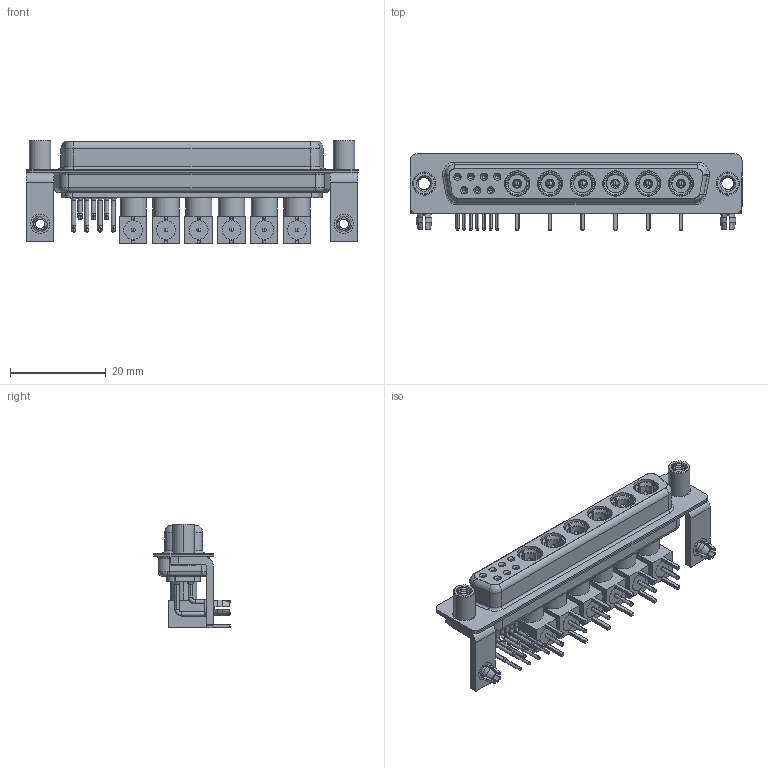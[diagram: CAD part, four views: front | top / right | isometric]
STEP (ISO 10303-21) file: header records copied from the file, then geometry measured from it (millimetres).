
FILE_DESCRIPTION (( 'STEP AP203' ), '1' );
FILE_NAME ('630-13W6240-7TD.STEP', '2022-06-03T13:02:00', ( '' ), ( '' ), 'SwSTEP 2.0', 'SolidWorks 2020', '' );
FILE_SCHEMA (( 'CONFIG_CONTROL_DESIGN' ));
Length unit declared in the file: millimetre
Products named in the file (21): Insulator RA Pin; RA Back Shell; 630Combo Contact Row 1; Pin_RA; 630Combo Shell Front_37 Contacts; Co-Ax Plug Assy_RA; Co-Ax Plug_RA PC Tail; 630Combo Shell Rear_37 Contacts; 630Combo Stabilizer Bracket; 630Combo Board Lock; Locking Collar; 630Combo Contact Row 2; 630Combo Housing_13W6; Insulator Pin_Straight PC Tail; 630Combo Threaded Standoff_D; 630-13W6240-7TD
Assembly tree (58 placements, depth 3):
  630-13W6240-7TD
    630Combo Housing_13W6
    630Combo Shell Front_37 Contacts
    630Combo Shell Rear_37 Contacts
    630Combo Stabilizer Bracket  x2
    630Combo Board Lock  x2
    630Combo Threaded Standoff_D  x2
    Co-Ax Plug Assy_RA
      Co-Ax Plug_RA PC Tail
      Insulator Pin_Straight PC Tail
      Pin_RA
      Locking Collar
      RA Back Shell
      Insulator RA Pin
    Co-Ax Plug Assy_RA
      Co-Ax Plug_RA PC Tail
      Insulator Pin_Straight PC Tail
      Pin_RA
      Locking Collar
      RA Back Shell
      Insulator RA Pin
    Co-Ax Plug Assy_RA
      Co-Ax Plug_RA PC Tail
      Insulator Pin_Straight PC Tail
      Pin_RA
      Locking Collar
      RA Back Shell
      Insulator RA Pin
    Co-Ax Plug Assy_RA
      Co-Ax Plug_RA PC Tail
      Insulator Pin_Straight PC Tail
      Pin_RA
      Locking Collar
      RA Back Shell
      Insulator RA Pin
    Co-Ax Plug Assy_RA
      Co-Ax Plug_RA PC Tail
      Insulator Pin_Straight PC Tail
      Pin_RA
      Locking Collar
      RA Back Shell
      Insulator RA Pin
    Co-Ax Plug Assy_RA
      Co-Ax Plug_RA PC Tail
      Insulator Pin_Straight PC Tail
      Pin_RA
      Locking Collar
      RA Back Shell
      Insulator RA Pin
    630Combo Contact Row 1  x4
    630Combo Contact Row 2  x3
Bounding box: 69.4 x 16 x 21.61 mm (x, y, z)
Volume: 7089.7 mm3; surface area: 17090.2 mm2
Topology: 52 solids, 52 shells, 1848 faces, 4550 edges, 2866 vertices
Faces by surface type: cylinder 792, plane 644, cone 255, torus 93, bspline 40, sphere 24
Entity records: 26930 total; most frequent: CARTESIAN_POINT 6550, DIRECTION 3872, ORIENTED_EDGE 3424, EDGE_CURVE 1712, AXIS2_PLACEMENT_3D 1570, VERTEX_POINT 1093, EDGE_LOOP 817, CIRCLE 810
